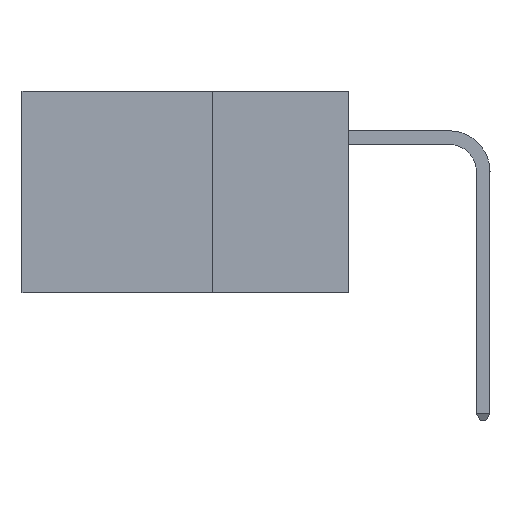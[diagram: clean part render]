
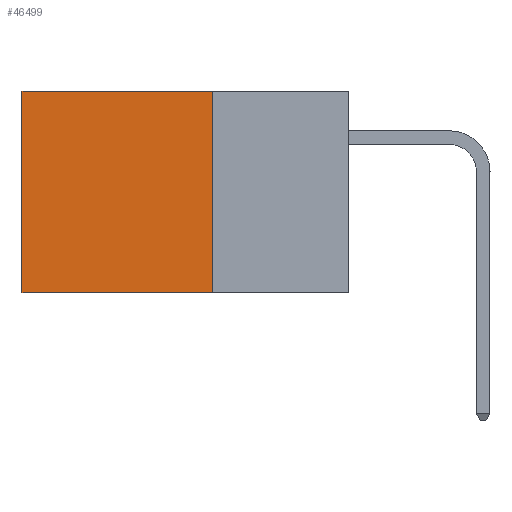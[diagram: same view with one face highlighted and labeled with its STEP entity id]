
A CAD part, left-side view. The second image highlights one B-rep face of the part: STEP entity #46499.
In plain terms, the highlighted planar face has unit normal (-1, 0, 0).
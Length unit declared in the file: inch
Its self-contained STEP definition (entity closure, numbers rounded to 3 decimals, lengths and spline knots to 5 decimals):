
#103 = CARTESIAN_POINT ( 'NONE',  ( 0.2875, 0.25, 0. ) ) ;
#428 = VERTEX_POINT ( 'NONE', #14927 ) ;
#1172 = CARTESIAN_POINT ( 'NONE',  ( 0.2875, 0.25, -0.37 ) ) ;
#2072 = VECTOR ( 'NONE', #14499, 39.37008 ) ;
#2643 = EDGE_CURVE ( 'NONE', #39107, #35573, #20471, .T. ) ;
#3131 = DIRECTION ( 'NONE',  ( 0., 0., -1. ) ) ;
#5652 = VECTOR ( 'NONE', #12391, 39.37008 ) ;
#7009 = VECTOR ( 'NONE', #41189, 39.37008 ) ;
#8799 = EDGE_LOOP ( 'NONE', ( #21956, #29802, #40364, #9762 ) ) ;
#9762 = ORIENTED_EDGE ( 'NONE', *, *, #2643, .T. ) ;
#10609 = PLANE ( 'NONE',  #46370 ) ;
#12391 = DIRECTION ( 'NONE',  ( 0., 1., 0. ) ) ;
#13081 = CARTESIAN_POINT ( 'NONE',  ( 0.2875, 0.25, 0. ) ) ;
#13920 = VERTEX_POINT ( 'NONE', #18899 ) ;
#14499 = DIRECTION ( 'NONE',  ( 0., 0., -1. ) ) ;
#14826 = DIRECTION ( 'NONE',  ( 0., 1., 0. ) ) ;
#14927 = CARTESIAN_POINT ( 'NONE',  ( 0.2875, 0.25, -0.37 ) ) ;
#16069 = LINE ( 'NONE', #30550, #7009 ) ;
#16737 = DIRECTION ( 'NONE',  ( 1., 0., 0. ) ) ;
#18899 = CARTESIAN_POINT ( 'NONE',  ( 0.2875, 0.6, -0.37 ) ) ;
#19771 = EDGE_CURVE ( 'NONE', #428, #13920, #44380, .T. ) ;
#20471 = LINE ( 'NONE', #103, #22214 ) ;
#21019 = CARTESIAN_POINT ( 'NONE',  ( 0.2875, 0.25, 0. ) ) ;
#21956 = ORIENTED_EDGE ( 'NONE', *, *, #44779, .T. ) ;
#22214 = VECTOR ( 'NONE', #14826, 39.37008 ) ;
#29802 = ORIENTED_EDGE ( 'NONE', *, *, #19771, .F. ) ;
#30550 = CARTESIAN_POINT ( 'NONE',  ( 0.2875, 0.25, 0. ) ) ;
#31168 = FACE_OUTER_BOUND ( 'NONE', #8799, .T. ) ;
#33177 = CARTESIAN_POINT ( 'NONE',  ( 0.2875, 0.6, 0. ) ) ;
#35573 = VERTEX_POINT ( 'NONE', #36280 ) ;
#35619 = LINE ( 'NONE', #33177, #2072 ) ;
#36280 = CARTESIAN_POINT ( 'NONE',  ( 0.2875, 0.6, 0. ) ) ;
#39107 = VERTEX_POINT ( 'NONE', #21019 ) ;
#40079 = EDGE_CURVE ( 'NONE', #39107, #428, #16069, .T. ) ;
#40364 = ORIENTED_EDGE ( 'NONE', *, *, #40079, .F. ) ;
#41189 = DIRECTION ( 'NONE',  ( 0., 0., -1. ) ) ;
#44380 = LINE ( 'NONE', #1172, #5652 ) ;
#44779 = EDGE_CURVE ( 'NONE', #35573, #13920, #35619, .T. ) ;
#46370 = AXIS2_PLACEMENT_3D ( 'NONE', #13081, #16737, #3131 ) ;
#46499 = ADVANCED_FACE ( 'NONE', ( #31168 ), #10609, .F. ) ;
